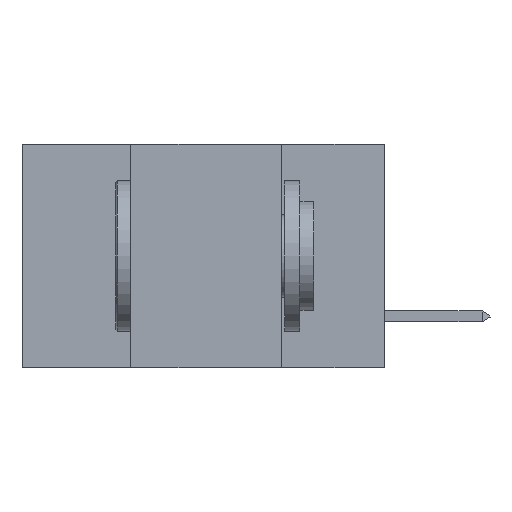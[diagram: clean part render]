
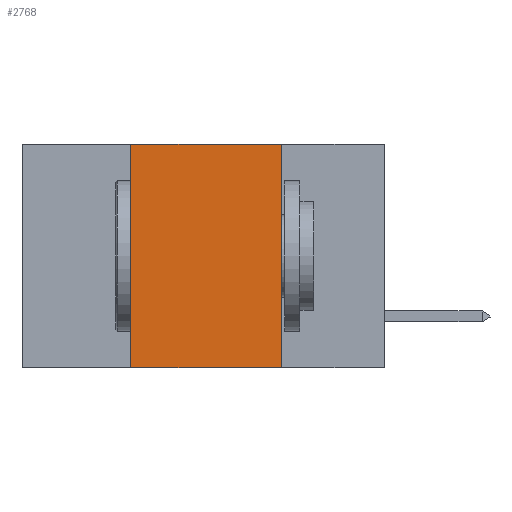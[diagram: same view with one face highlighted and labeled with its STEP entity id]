
A CAD part, left-side view. The second image highlights one B-rep face of the part: STEP entity #2768.
In plain terms, the highlighted planar face has unit normal (-1, 0, 0).
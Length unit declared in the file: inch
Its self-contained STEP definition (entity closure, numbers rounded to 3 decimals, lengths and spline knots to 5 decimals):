
#2063 = CARTESIAN_POINT ( 'NONE',  ( 0., 0.6, -0.37 ) ) ;
#2127 = VECTOR ( 'NONE', #7046, 39.37008 ) ;
#2135 = VERTEX_POINT ( 'NONE', #43936 ) ;
#2768 = ADVANCED_FACE ( 'NONE', ( #36895 ), #45401, .F. ) ;
#4621 = ORIENTED_EDGE ( 'NONE', *, *, #6560, .F. ) ;
#5408 = EDGE_CURVE ( 'NONE', #17119, #38019, #36558, .T. ) ;
#6560 = EDGE_CURVE ( 'NONE', #2135, #17119, #6883, .T. ) ;
#6617 = VERTEX_POINT ( 'NONE', #38669 ) ;
#6883 = LINE ( 'NONE', #22694, #46055 ) ;
#7046 = DIRECTION ( 'NONE',  ( 0., -1., 0. ) ) ;
#7565 = VECTOR ( 'NONE', #46878, 39.37008 ) ;
#7941 = DIRECTION ( 'NONE',  ( 1., 0., 0. ) ) ;
#9870 = ORIENTED_EDGE ( 'NONE', *, *, #5408, .F. ) ;
#11035 = VECTOR ( 'NONE', #12959, 39.37008 ) ;
#11440 = DIRECTION ( 'NONE',  ( 0., 0., -1. ) ) ;
#12267 = LINE ( 'NONE', #2063, #2127 ) ;
#12959 = DIRECTION ( 'NONE',  ( 0., -1., 0. ) ) ;
#16936 = ORIENTED_EDGE ( 'NONE', *, *, #27789, .T. ) ;
#17119 = VERTEX_POINT ( 'NONE', #30998 ) ;
#17226 = EDGE_CURVE ( 'NONE', #38019, #6617, #32501, .T. ) ;
#19141 = EDGE_LOOP ( 'NONE', ( #43270, #9870, #4621, #16936 ) ) ;
#22694 = CARTESIAN_POINT ( 'NONE',  ( 0., 0.42, 0. ) ) ;
#27467 = DIRECTION ( 'NONE',  ( 0., 0., 1. ) ) ;
#27789 = EDGE_CURVE ( 'NONE', #2135, #6617, #12267, .T. ) ;
#28343 = CARTESIAN_POINT ( 'NONE',  ( 0., 0.17, 0. ) ) ;
#30998 = CARTESIAN_POINT ( 'NONE',  ( 0., 0.42, 0. ) ) ;
#31573 = AXIS2_PLACEMENT_3D ( 'NONE', #42237, #7941, #11440 ) ;
#32501 = LINE ( 'NONE', #39592, #7565 ) ;
#36558 = LINE ( 'NONE', #43260, #11035 ) ;
#36895 = FACE_OUTER_BOUND ( 'NONE', #19141, .T. ) ;
#38019 = VERTEX_POINT ( 'NONE', #28343 ) ;
#38669 = CARTESIAN_POINT ( 'NONE',  ( 0., 0.17, -0.37 ) ) ;
#39592 = CARTESIAN_POINT ( 'NONE',  ( 0., 0.17, 0. ) ) ;
#42237 = CARTESIAN_POINT ( 'NONE',  ( 0., 0.6, 0. ) ) ;
#43260 = CARTESIAN_POINT ( 'NONE',  ( 0., 0.6, 0. ) ) ;
#43270 = ORIENTED_EDGE ( 'NONE', *, *, #17226, .F. ) ;
#43936 = CARTESIAN_POINT ( 'NONE',  ( 0., 0.42, -0.37 ) ) ;
#45401 = PLANE ( 'NONE',  #31573 ) ;
#46055 = VECTOR ( 'NONE', #27467, 39.37008 ) ;
#46878 = DIRECTION ( 'NONE',  ( 0., 0., -1. ) ) ;
